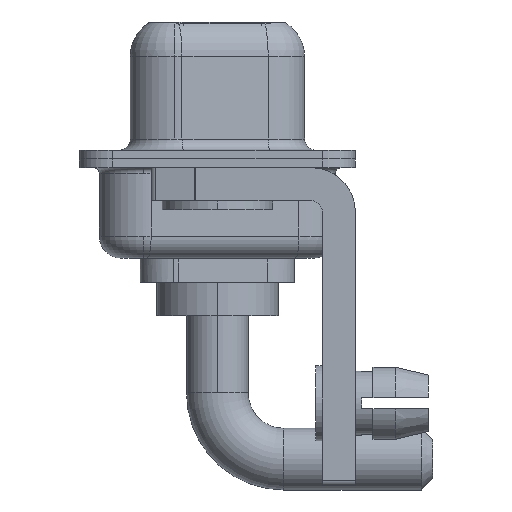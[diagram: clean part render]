
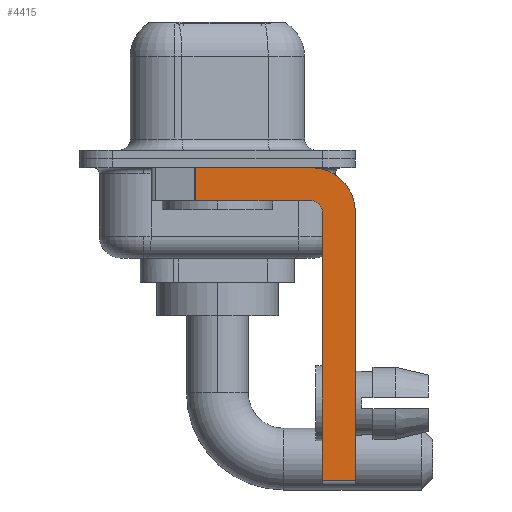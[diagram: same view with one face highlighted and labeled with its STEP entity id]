
A CAD part, left-side view. The second image highlights one B-rep face of the part: STEP entity #4415.
In plain terms, the highlighted planar face has unit normal (-1, 0, 0).
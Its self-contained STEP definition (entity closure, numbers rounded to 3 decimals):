
#495 = CARTESIAN_POINT ( 'NONE',  ( -2.9, -4.25, -0.4 ) ) ;
#1012 = DIRECTION ( 'NONE',  ( 0., -1., 0. ) ) ;
#1364 = DIRECTION ( 'NONE',  ( -1., 0., 0. ) ) ;
#1412 = DIRECTION ( 'NONE',  ( 0., 0., -1. ) ) ;
#1427 = VERTEX_POINT ( 'NONE', #14137 ) ;
#1562 = ORIENTED_EDGE ( 'NONE', *, *, #4696, .F. ) ;
#1678 = CARTESIAN_POINT ( 'NONE',  ( -2.9, -4.25, -14.55 ) ) ;
#2003 = DIRECTION ( 'NONE',  ( 0., 1., 0. ) ) ;
#2156 = CARTESIAN_POINT ( 'NONE',  ( -2.9, -4.25, -1.9 ) ) ;
#2226 = VERTEX_POINT ( 'NONE', #14487 ) ;
#2540 = CIRCLE ( 'NONE', #8406, 2. ) ;
#2582 = LINE ( 'NONE', #10300, #4320 ) ;
#3082 = VERTEX_POINT ( 'NONE', #14507 ) ;
#3873 = PLANE ( 'NONE',  #10839 ) ;
#3941 = DIRECTION ( 'NONE',  ( 0., 0., -1. ) ) ;
#4109 = VERTEX_POINT ( 'NONE', #12274 ) ;
#4206 = ORIENTED_EDGE ( 'NONE', *, *, #7411, .F. ) ;
#4320 = VECTOR ( 'NONE', #1412, 1000. ) ;
#4415 = ADVANCED_FACE ( 'NONE', ( #9460 ), #3873, .F. ) ;
#4696 = EDGE_CURVE ( 'NONE', #6653, #1427, #7082, .T. ) ;
#4950 = DIRECTION ( 'NONE',  ( 0., 0., -1. ) ) ;
#5535 = VECTOR ( 'NONE', #1012, 1000. ) ;
#5834 = LINE ( 'NONE', #10318, #5968 ) ;
#5968 = VECTOR ( 'NONE', #9219, 1000. ) ;
#6079 = ORIENTED_EDGE ( 'NONE', *, *, #11274, .T. ) ;
#6653 = VERTEX_POINT ( 'NONE', #10855 ) ;
#7010 = CARTESIAN_POINT ( 'NONE',  ( -2.9, -6.25, -2.4 ) ) ;
#7082 = CIRCLE ( 'NONE', #10139, 0.5 ) ;
#7411 = EDGE_CURVE ( 'NONE', #4109, #6653, #5834, .T. ) ;
#7555 = DIRECTION ( 'NONE',  ( 1., 0., 0. ) ) ;
#7586 = LINE ( 'NONE', #2156, #9984 ) ;
#7694 = EDGE_CURVE ( 'NONE', #1427, #3082, #7586, .T. ) ;
#7725 = CARTESIAN_POINT ( 'NONE',  ( -2.9, -6.25, -2.4 ) ) ;
#8114 = ORIENTED_EDGE ( 'NONE', *, *, #13323, .F. ) ;
#8406 = AXIS2_PLACEMENT_3D ( 'NONE', #13362, #7555, #8659 ) ;
#8493 = VERTEX_POINT ( 'NONE', #495 ) ;
#8659 = DIRECTION ( 'NONE',  ( 0., 0., -1. ) ) ;
#9079 = VECTOR ( 'NONE', #13800, 1000. ) ;
#9219 = DIRECTION ( 'NONE',  ( 0., 0., 1. ) ) ;
#9231 = CARTESIAN_POINT ( 'NONE',  ( -2.9, -4.25, -2.4 ) ) ;
#9320 = LINE ( 'NONE', #1678, #9079 ) ;
#9460 = FACE_OUTER_BOUND ( 'NONE', #14521, .T. ) ;
#9768 = ORIENTED_EDGE ( 'NONE', *, *, #11554, .F. ) ;
#9984 = VECTOR ( 'NONE', #2003, 1000. ) ;
#10046 = DIRECTION ( 'NONE',  ( 0., 0., 1. ) ) ;
#10139 = AXIS2_PLACEMENT_3D ( 'NONE', #9231, #1364, #10046 ) ;
#10300 = CARTESIAN_POINT ( 'NONE',  ( -2.9, 0.978, -1.9 ) ) ;
#10318 = CARTESIAN_POINT ( 'NONE',  ( -2.9, -4.75, -14.8 ) ) ;
#10386 = VERTEX_POINT ( 'NONE', #13353 ) ;
#10436 = EDGE_CURVE ( 'NONE', #10386, #8493, #11002, .T. ) ;
#10518 = ORIENTED_EDGE ( 'NONE', *, *, #12000, .T. ) ;
#10839 = AXIS2_PLACEMENT_3D ( 'NONE', #12837, #14005, #3941 ) ;
#10855 = CARTESIAN_POINT ( 'NONE',  ( -2.9, -4.75, -2.4 ) ) ;
#11002 = LINE ( 'NONE', #14457, #5535 ) ;
#11274 = EDGE_CURVE ( 'NONE', #4109, #2226, #9320, .T. ) ;
#11554 = EDGE_CURVE ( 'NONE', #14092, #2226, #13844, .T. ) ;
#11926 = VECTOR ( 'NONE', #4950, 1000. ) ;
#12000 = EDGE_CURVE ( 'NONE', #10386, #3082, #2582, .T. ) ;
#12049 = ORIENTED_EDGE ( 'NONE', *, *, #10436, .F. ) ;
#12274 = CARTESIAN_POINT ( 'NONE',  ( -2.9, -4.75, -14.55 ) ) ;
#12837 = CARTESIAN_POINT ( 'NONE',  ( -2.9, -4.25, -2.4 ) ) ;
#13323 = EDGE_CURVE ( 'NONE', #8493, #14092, #2540, .T. ) ;
#13353 = CARTESIAN_POINT ( 'NONE',  ( -2.9, 0.978, -0.4 ) ) ;
#13362 = CARTESIAN_POINT ( 'NONE',  ( -2.9, -4.25, -2.4 ) ) ;
#13800 = DIRECTION ( 'NONE',  ( 0., -1., 0. ) ) ;
#13844 = LINE ( 'NONE', #7010, #11926 ) ;
#14005 = DIRECTION ( 'NONE',  ( 1., 0., 0. ) ) ;
#14092 = VERTEX_POINT ( 'NONE', #7725 ) ;
#14137 = CARTESIAN_POINT ( 'NONE',  ( -2.9, -4.25, -1.9 ) ) ;
#14457 = CARTESIAN_POINT ( 'NONE',  ( -2.9, 3., -0.4 ) ) ;
#14487 = CARTESIAN_POINT ( 'NONE',  ( -2.9, -6.25, -14.55 ) ) ;
#14507 = CARTESIAN_POINT ( 'NONE',  ( -2.9, 0.978, -1.9 ) ) ;
#14511 = ORIENTED_EDGE ( 'NONE', *, *, #7694, .F. ) ;
#14521 = EDGE_LOOP ( 'NONE', ( #12049, #10518, #14511, #1562, #4206, #6079, #9768, #8114 ) ) ;
